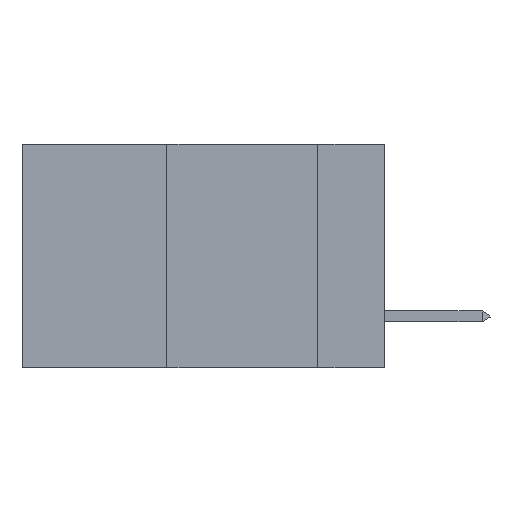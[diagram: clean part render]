
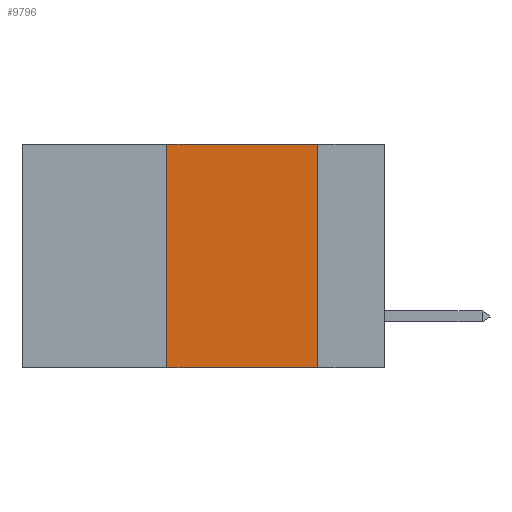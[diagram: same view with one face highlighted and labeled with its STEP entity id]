
A CAD part, left-side view. The second image highlights one B-rep face of the part: STEP entity #9796.
In plain terms, the highlighted planar face has unit normal (-1, 0, 0).
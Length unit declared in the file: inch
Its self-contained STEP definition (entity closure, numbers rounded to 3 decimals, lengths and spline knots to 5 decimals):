
#102 = DIRECTION ( 'NONE',  ( 1., 0., 0. ) ) ;
#525 = CARTESIAN_POINT ( 'NONE',  ( 0., 0.36, 0. ) ) ;
#1498 = VERTEX_POINT ( 'NONE', #1951 ) ;
#1696 = EDGE_LOOP ( 'NONE', ( #4021, #9979, #9492, #6830 ) ) ;
#1800 = CARTESIAN_POINT ( 'NONE',  ( 0., 0.36, -0.37 ) ) ;
#1951 = CARTESIAN_POINT ( 'NONE',  ( 0., 0.11, 0. ) ) ;
#2089 = EDGE_CURVE ( 'NONE', #8447, #2980, #4577, .T. ) ;
#2449 = CARTESIAN_POINT ( 'NONE',  ( 0., 0.11, -0.37 ) ) ;
#2523 = PLANE ( 'NONE',  #10649 ) ;
#2711 = LINE ( 'NONE', #7887, #6182 ) ;
#2773 = VERTEX_POINT ( 'NONE', #2449 ) ;
#2789 = CARTESIAN_POINT ( 'NONE',  ( 0., 0.6, 0. ) ) ;
#2980 = VERTEX_POINT ( 'NONE', #10728 ) ;
#3412 = EDGE_CURVE ( 'NONE', #2980, #1498, #9252, .T. ) ;
#4021 = ORIENTED_EDGE ( 'NONE', *, *, #5066, .F. ) ;
#4577 = LINE ( 'NONE', #525, #6658 ) ;
#5066 = EDGE_CURVE ( 'NONE', #1498, #2773, #2711, .T. ) ;
#5233 = DIRECTION ( 'NONE',  ( 0., 0., -1. ) ) ;
#5753 = DIRECTION ( 'NONE',  ( 0., -1., 0. ) ) ;
#6038 = CARTESIAN_POINT ( 'NONE',  ( 0., 0.6, -0.37 ) ) ;
#6079 = EDGE_CURVE ( 'NONE', #8447, #2773, #8925, .T. ) ;
#6182 = VECTOR ( 'NONE', #5233, 39.37008 ) ;
#6658 = VECTOR ( 'NONE', #11168, 39.37008 ) ;
#6830 = ORIENTED_EDGE ( 'NONE', *, *, #6079, .T. ) ;
#7887 = CARTESIAN_POINT ( 'NONE',  ( 0., 0.11, 0. ) ) ;
#8447 = VERTEX_POINT ( 'NONE', #1800 ) ;
#8678 = CARTESIAN_POINT ( 'NONE',  ( 0., 0.6, 0. ) ) ;
#8925 = LINE ( 'NONE', #6038, #9191 ) ;
#8941 = DIRECTION ( 'NONE',  ( 0., -1., 0. ) ) ;
#9191 = VECTOR ( 'NONE', #5753, 39.37008 ) ;
#9252 = LINE ( 'NONE', #2789, #11042 ) ;
#9492 = ORIENTED_EDGE ( 'NONE', *, *, #2089, .F. ) ;
#9796 = ADVANCED_FACE ( 'NONE', ( #10196 ), #2523, .F. ) ;
#9819 = DIRECTION ( 'NONE',  ( 0., 0., -1. ) ) ;
#9979 = ORIENTED_EDGE ( 'NONE', *, *, #3412, .F. ) ;
#10196 = FACE_OUTER_BOUND ( 'NONE', #1696, .T. ) ;
#10649 = AXIS2_PLACEMENT_3D ( 'NONE', #8678, #102, #9819 ) ;
#10728 = CARTESIAN_POINT ( 'NONE',  ( 0., 0.36, 0. ) ) ;
#11042 = VECTOR ( 'NONE', #8941, 39.37008 ) ;
#11168 = DIRECTION ( 'NONE',  ( 0., 0., 1. ) ) ;
